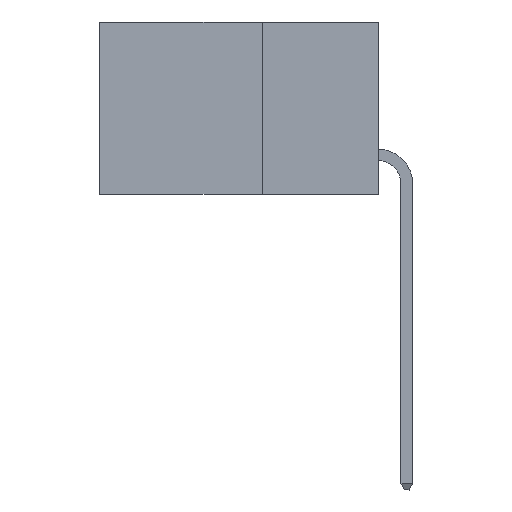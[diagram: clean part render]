
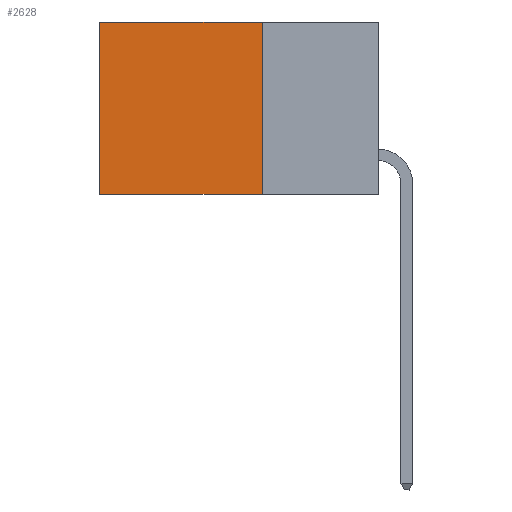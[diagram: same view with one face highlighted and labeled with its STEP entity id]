
A CAD part, left-side view. The second image highlights one B-rep face of the part: STEP entity #2628.
In plain terms, the highlighted planar face has unit normal (-1, 0, 0).
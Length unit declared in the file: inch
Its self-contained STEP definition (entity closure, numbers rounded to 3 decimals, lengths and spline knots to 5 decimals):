
#24 = VECTOR ( 'NONE', #7893, 39.37008 ) ;
#112 = VECTOR ( 'NONE', #366, 39.37008 ) ;
#366 = DIRECTION ( 'NONE',  ( 0., 0., -1. ) ) ;
#733 = CARTESIAN_POINT ( 'NONE',  ( 0.298, 0.25, 0. ) ) ;
#1038 = EDGE_CURVE ( 'NONE', #12427, #9059, #8403, .T. ) ;
#1069 = CARTESIAN_POINT ( 'NONE',  ( 0.298, 0.25, 0. ) ) ;
#1470 = DIRECTION ( 'NONE',  ( 0., 0., -1. ) ) ;
#1485 = ORIENTED_EDGE ( 'NONE', *, *, #1038, .T. ) ;
#1599 = DIRECTION ( 'NONE',  ( 0., 0., -1. ) ) ;
#1612 = DIRECTION ( 'NONE',  ( 1., 0., 0. ) ) ;
#2152 = LINE ( 'NONE', #6363, #112 ) ;
#2628 = ADVANCED_FACE ( 'NONE', ( #4790 ), #10115, .F. ) ;
#3110 = VECTOR ( 'NONE', #1470, 39.37008 ) ;
#3322 = VECTOR ( 'NONE', #6063, 39.37008 ) ;
#3666 = LINE ( 'NONE', #1069, #3322 ) ;
#4773 = CARTESIAN_POINT ( 'NONE',  ( 0.298, 0.25, 0. ) ) ;
#4790 = FACE_OUTER_BOUND ( 'NONE', #8319, .T. ) ;
#6063 = DIRECTION ( 'NONE',  ( 0., 1., 0. ) ) ;
#6363 = CARTESIAN_POINT ( 'NONE',  ( 0.298, 0.25, 0. ) ) ;
#6673 = AXIS2_PLACEMENT_3D ( 'NONE', #733, #1612, #1599 ) ;
#6875 = CARTESIAN_POINT ( 'NONE',  ( 0.298, 0.25, -0.37 ) ) ;
#7386 = VERTEX_POINT ( 'NONE', #4773 ) ;
#7893 = DIRECTION ( 'NONE',  ( 0., 1., 0. ) ) ;
#8020 = LINE ( 'NONE', #6875, #24 ) ;
#8103 = CARTESIAN_POINT ( 'NONE',  ( 0.298, 0.6, 0. ) ) ;
#8319 = EDGE_LOOP ( 'NONE', ( #1485, #9466, #12091, #12374 ) ) ;
#8403 = LINE ( 'NONE', #11702, #3110 ) ;
#9059 = VERTEX_POINT ( 'NONE', #12582 ) ;
#9466 = ORIENTED_EDGE ( 'NONE', *, *, #10327, .F. ) ;
#9688 = CARTESIAN_POINT ( 'NONE',  ( 0.298, 0.25, -0.37 ) ) ;
#10115 = PLANE ( 'NONE',  #6673 ) ;
#10327 = EDGE_CURVE ( 'NONE', #10578, #9059, #8020, .T. ) ;
#10578 = VERTEX_POINT ( 'NONE', #9688 ) ;
#10636 = EDGE_CURVE ( 'NONE', #7386, #12427, #3666, .T. ) ;
#11487 = EDGE_CURVE ( 'NONE', #7386, #10578, #2152, .T. ) ;
#11702 = CARTESIAN_POINT ( 'NONE',  ( 0.298, 0.6, 0. ) ) ;
#12091 = ORIENTED_EDGE ( 'NONE', *, *, #11487, .F. ) ;
#12374 = ORIENTED_EDGE ( 'NONE', *, *, #10636, .T. ) ;
#12427 = VERTEX_POINT ( 'NONE', #8103 ) ;
#12582 = CARTESIAN_POINT ( 'NONE',  ( 0.298, 0.6, -0.37 ) ) ;
